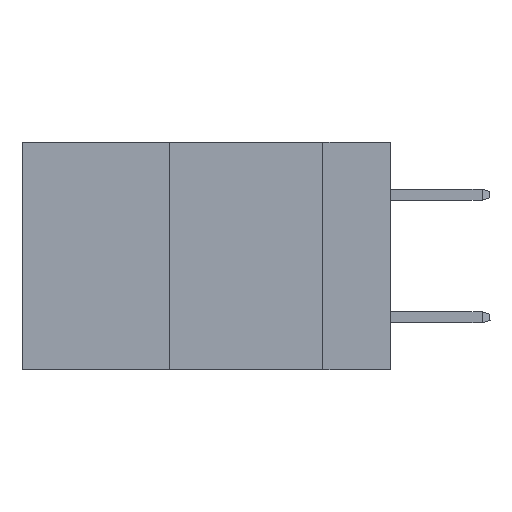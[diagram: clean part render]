
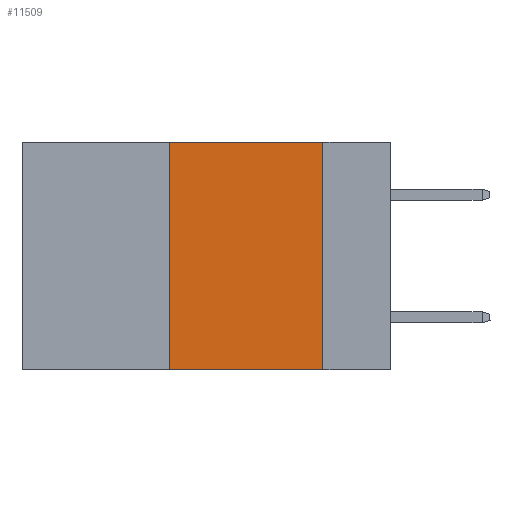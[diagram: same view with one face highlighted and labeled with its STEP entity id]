
A CAD part, left-side view. The second image highlights one B-rep face of the part: STEP entity #11509.
In plain terms, the highlighted planar face has unit normal (-1, 0, 0).
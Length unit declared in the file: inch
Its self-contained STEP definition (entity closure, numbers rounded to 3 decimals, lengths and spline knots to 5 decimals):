
#412 = CARTESIAN_POINT ( 'NONE',  ( 0., 0.11, -0.37 ) ) ;
#415 = PLANE ( 'NONE',  #1531 ) ;
#569 = FACE_OUTER_BOUND ( 'NONE', #2048, .T. ) ;
#852 = CARTESIAN_POINT ( 'NONE',  ( 0., 0.36, 0. ) ) ;
#869 = CARTESIAN_POINT ( 'NONE',  ( 0., 0.11, 0. ) ) ;
#1521 = DIRECTION ( 'NONE',  ( 1., 0., 0. ) ) ;
#1531 = AXIS2_PLACEMENT_3D ( 'NONE', #11954, #1521, #8898 ) ;
#1959 = VERTEX_POINT ( 'NONE', #10405 ) ;
#2048 = EDGE_LOOP ( 'NONE', ( #13322, #5343, #8168, #10925 ) ) ;
#2736 = VECTOR ( 'NONE', #3519, 39.37008 ) ;
#3519 = DIRECTION ( 'NONE',  ( 0., -1., 0. ) ) ;
#3854 = LINE ( 'NONE', #9050, #6960 ) ;
#3978 = EDGE_CURVE ( 'NONE', #1959, #4061, #5505, .T. ) ;
#4061 = VERTEX_POINT ( 'NONE', #412 ) ;
#5343 = ORIENTED_EDGE ( 'NONE', *, *, #9020, .F. ) ;
#5505 = LINE ( 'NONE', #8761, #2736 ) ;
#6070 = EDGE_CURVE ( 'NONE', #1959, #6912, #3854, .T. ) ;
#6119 = LINE ( 'NONE', #11418, #11990 ) ;
#6912 = VERTEX_POINT ( 'NONE', #852 ) ;
#6960 = VECTOR ( 'NONE', #12111, 39.37008 ) ;
#7026 = DIRECTION ( 'NONE',  ( 0., 0., -1. ) ) ;
#7484 = EDGE_CURVE ( 'NONE', #9626, #4061, #11168, .T. ) ;
#8168 = ORIENTED_EDGE ( 'NONE', *, *, #6070, .F. ) ;
#8403 = VECTOR ( 'NONE', #7026, 39.37008 ) ;
#8761 = CARTESIAN_POINT ( 'NONE',  ( 0., 0.6, -0.37 ) ) ;
#8898 = DIRECTION ( 'NONE',  ( 0., 0., -1. ) ) ;
#9020 = EDGE_CURVE ( 'NONE', #6912, #9626, #6119, .T. ) ;
#9050 = CARTESIAN_POINT ( 'NONE',  ( 0., 0.36, 0. ) ) ;
#9626 = VERTEX_POINT ( 'NONE', #869 ) ;
#10405 = CARTESIAN_POINT ( 'NONE',  ( 0., 0.36, -0.37 ) ) ;
#10925 = ORIENTED_EDGE ( 'NONE', *, *, #3978, .T. ) ;
#11168 = LINE ( 'NONE', #12212, #8403 ) ;
#11418 = CARTESIAN_POINT ( 'NONE',  ( 0., 0.6, 0. ) ) ;
#11509 = ADVANCED_FACE ( 'NONE', ( #569 ), #415, .F. ) ;
#11954 = CARTESIAN_POINT ( 'NONE',  ( 0., 0.6, 0. ) ) ;
#11990 = VECTOR ( 'NONE', #12442, 39.37008 ) ;
#12111 = DIRECTION ( 'NONE',  ( 0., 0., 1. ) ) ;
#12212 = CARTESIAN_POINT ( 'NONE',  ( 0., 0.11, 0. ) ) ;
#12442 = DIRECTION ( 'NONE',  ( 0., -1., 0. ) ) ;
#13322 = ORIENTED_EDGE ( 'NONE', *, *, #7484, .F. ) ;
